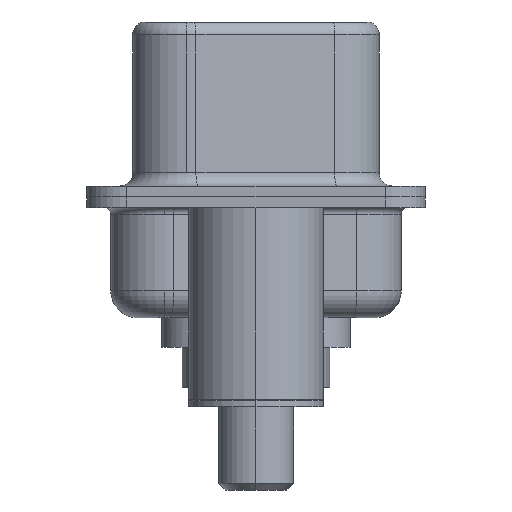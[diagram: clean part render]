
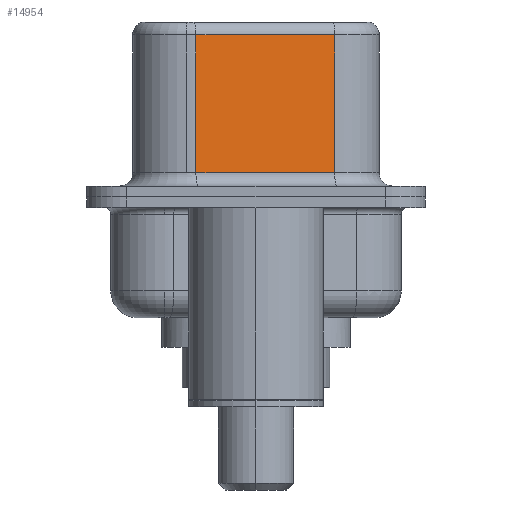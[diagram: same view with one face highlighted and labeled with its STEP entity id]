
A CAD part, left-side view. The second image highlights one B-rep face of the part: STEP entity #14954.
In plain terms, the highlighted planar face has unit normal (-0.985, -0.174, 0).
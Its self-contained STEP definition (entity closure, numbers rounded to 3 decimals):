
#165 = EDGE_LOOP ( 'NONE', ( #3501, #10216, #6607, #13682 ) ) ;
#296 = EDGE_CURVE ( 'NONE', #2009, #12446, #5278, .T. ) ;
#573 = EDGE_CURVE ( 'NONE', #5240, #9575, #14248, .T. ) ;
#815 = CARTESIAN_POINT ( 'NONE',  ( 4.565, -2.927, 6.52 ) ) ;
#1374 = FACE_OUTER_BOUND ( 'NONE', #165, .T. ) ;
#1943 = DIRECTION ( 'NONE',  ( 0.174, -0.985, 0. ) ) ;
#2009 = VERTEX_POINT ( 'NONE', #15019 ) ;
#2778 = CARTESIAN_POINT ( 'NONE',  ( 4.565, -2.927, 0.9 ) ) ;
#2979 = PLANE ( 'NONE',  #9587 ) ;
#3033 = CARTESIAN_POINT ( 'NONE',  ( 4.565, -2.927, 6.52 ) ) ;
#3501 = ORIENTED_EDGE ( 'NONE', *, *, #296, .F. ) ;
#4079 = EDGE_CURVE ( 'NONE', #9575, #12446, #5427, .T. ) ;
#5240 = VERTEX_POINT ( 'NONE', #15092 ) ;
#5278 = LINE ( 'NONE', #815, #15494 ) ;
#5427 = LINE ( 'NONE', #7027, #15637 ) ;
#5518 = VECTOR ( 'NONE', #8413, 1000. ) ;
#5687 = DIRECTION ( 'NONE',  ( 0.985, 0.174, 0. ) ) ;
#6607 = ORIENTED_EDGE ( 'NONE', *, *, #573, .T. ) ;
#7027 = CARTESIAN_POINT ( 'NONE',  ( 4.565, -2.927, 0.9 ) ) ;
#7493 = DIRECTION ( 'NONE',  ( 0., 0., -1. ) ) ;
#7806 = CARTESIAN_POINT ( 'NONE',  ( 3.655, 2.233, 0.9 ) ) ;
#8413 = DIRECTION ( 'NONE',  ( -0.174, 0.985, 0. ) ) ;
#9120 = EDGE_CURVE ( 'NONE', #2009, #5240, #16560, .T. ) ;
#9575 = VERTEX_POINT ( 'NONE', #7806 ) ;
#9587 = AXIS2_PLACEMENT_3D ( 'NONE', #3033, #5687, #15036 ) ;
#10216 = ORIENTED_EDGE ( 'NONE', *, *, #9120, .T. ) ;
#10974 = CARTESIAN_POINT ( 'NONE',  ( 4.565, -2.927, 6.02 ) ) ;
#11693 = CARTESIAN_POINT ( 'NONE',  ( 3.655, 2.233, 6.52 ) ) ;
#12446 = VERTEX_POINT ( 'NONE', #2778 ) ;
#13682 = ORIENTED_EDGE ( 'NONE', *, *, #4079, .T. ) ;
#14248 = LINE ( 'NONE', #11693, #15698 ) ;
#14954 = ADVANCED_FACE ( 'NONE', ( #1374 ), #2979, .F. ) ;
#15019 = CARTESIAN_POINT ( 'NONE',  ( 4.565, -2.927, 6.02 ) ) ;
#15036 = DIRECTION ( 'NONE',  ( -0.174, 0.985, 0. ) ) ;
#15092 = CARTESIAN_POINT ( 'NONE',  ( 3.655, 2.233, 6.02 ) ) ;
#15494 = VECTOR ( 'NONE', #15680, 1000. ) ;
#15637 = VECTOR ( 'NONE', #1943, 1000. ) ;
#15680 = DIRECTION ( 'NONE',  ( 0., 0., -1. ) ) ;
#15698 = VECTOR ( 'NONE', #7493, 1000. ) ;
#16560 = LINE ( 'NONE', #10974, #5518 ) ;
